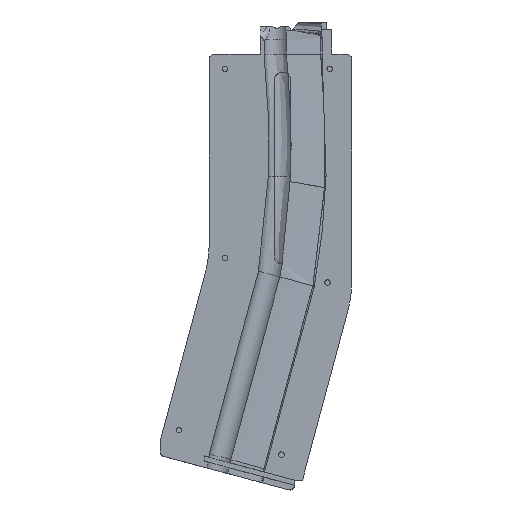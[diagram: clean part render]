
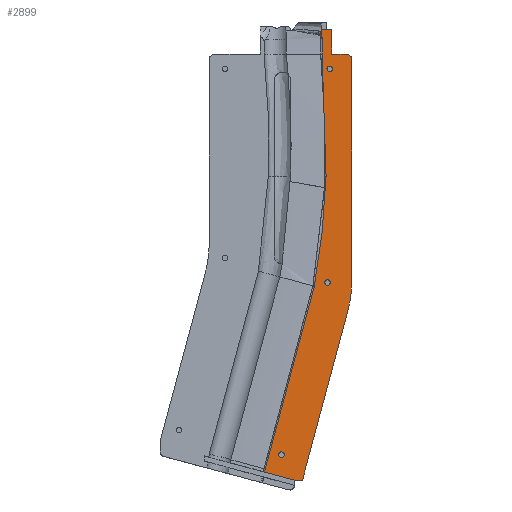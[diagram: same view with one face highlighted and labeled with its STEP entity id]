
A CAD part, front view. The second image highlights one B-rep face of the part: STEP entity #2899.
In plain terms, the highlighted planar face has unit normal (0, -1, 0).
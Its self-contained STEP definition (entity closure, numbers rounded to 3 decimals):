
#31=FACE_BOUND('',#755,.T.);
#32=FACE_BOUND('',#756,.T.);
#33=FACE_BOUND('',#757,.T.);
#140=LINE('',#5888,#327);
#141=LINE('',#5890,#328);
#142=LINE('',#5892,#329);
#143=LINE('',#5896,#330);
#144=LINE('',#5908,#331);
#145=LINE('',#5910,#332);
#146=LINE('',#5919,#333);
#147=LINE('',#5921,#334);
#148=LINE('',#5923,#335);
#149=LINE('',#5925,#336);
#150=LINE('',#5929,#337);
#151=LINE('',#5932,#338);
#327=VECTOR('',#3531,10.);
#328=VECTOR('',#3532,10.);
#329=VECTOR('',#3533,10.);
#330=VECTOR('',#3536,10.);
#331=VECTOR('',#3537,10.);
#332=VECTOR('',#3538,10.);
#333=VECTOR('',#3539,10.);
#334=VECTOR('',#3540,10.);
#335=VECTOR('',#3541,10.);
#336=VECTOR('',#3542,10.);
#337=VECTOR('',#3545,10.);
#338=VECTOR('',#3548,10.);
#470=PLANE('',#3127);
#571=FACE_OUTER_BOUND('',#754,.T.);
#754=EDGE_LOOP('',(#2173,#2174,#2175,#2176,#2177,#2178,#2179,#2180,#2181,
#2182,#2183,#2184,#2185,#2186,#2187,#2188,#2189,#2190));
#755=EDGE_LOOP('',(#2191));
#756=EDGE_LOOP('',(#2192));
#757=EDGE_LOOP('',(#2193));
#900=CIRCLE('',#3072,1.25);
#921=CIRCLE('',#3128,2.);
#922=CIRCLE('',#3129,50.);
#923=CIRCLE('',#3130,2.5);
#924=CIRCLE('',#3131,1.25);
#925=CIRCLE('',#3132,1.25);
#1108=B_SPLINE_CURVE_WITH_KNOTS('',3,(#5898,#5899,#5900,#5901),
 .UNSPECIFIED.,.F.,.F.,(4,4),(-5.507,0.),.UNSPECIFIED.);
#1109=B_SPLINE_CURVE_WITH_KNOTS('',3,(#5903,#5904,#5905,#5906),
 .UNSPECIFIED.,.F.,.F.,(4,4),(-4.958,0.),.UNSPECIFIED.);
#1110=B_SPLINE_CURVE_WITH_KNOTS('',3,(#5912,#5913,#5914,#5915,#5916,#5917),
 .UNSPECIFIED.,.F.,.F.,(4,2,4),(-0.151,-0.075,
0.),.UNSPECIFIED.);
#1230=VERTEX_POINT('',#5105);
#1302=VERTEX_POINT('',#5886);
#1303=VERTEX_POINT('',#5887);
#1304=VERTEX_POINT('',#5889);
#1305=VERTEX_POINT('',#5891);
#1306=VERTEX_POINT('',#5893);
#1307=VERTEX_POINT('',#5895);
#1308=VERTEX_POINT('',#5897);
#1309=VERTEX_POINT('',#5902);
#1310=VERTEX_POINT('',#5907);
#1311=VERTEX_POINT('',#5909);
#1312=VERTEX_POINT('',#5911);
#1313=VERTEX_POINT('',#5918);
#1314=VERTEX_POINT('',#5920);
#1315=VERTEX_POINT('',#5922);
#1316=VERTEX_POINT('',#5924);
#1317=VERTEX_POINT('',#5926);
#1318=VERTEX_POINT('',#5928);
#1319=VERTEX_POINT('',#5930);
#1320=VERTEX_POINT('',#5933);
#1321=VERTEX_POINT('',#5935);
#1531=EDGE_CURVE('',#1230,#1230,#900,.T.);
#1633=EDGE_CURVE('',#1302,#1303,#140,.T.);
#1634=EDGE_CURVE('',#1304,#1302,#141,.T.);
#1635=EDGE_CURVE('',#1305,#1304,#142,.T.);
#1636=EDGE_CURVE('',#1306,#1305,#921,.T.);
#1637=EDGE_CURVE('',#1307,#1306,#143,.T.);
#1638=EDGE_CURVE('',#1308,#1307,#1108,.T.);
#1639=EDGE_CURVE('',#1309,#1308,#1109,.T.);
#1640=EDGE_CURVE('',#1309,#1310,#144,.T.);
#1641=EDGE_CURVE('',#1310,#1311,#145,.T.);
#1642=EDGE_CURVE('',#1312,#1311,#1110,.T.);
#1643=EDGE_CURVE('',#1313,#1312,#146,.T.);
#1644=EDGE_CURVE('',#1314,#1313,#147,.T.);
#1645=EDGE_CURVE('',#1315,#1314,#148,.T.);
#1646=EDGE_CURVE('',#1315,#1316,#149,.T.);
#1647=EDGE_CURVE('',#1317,#1316,#922,.F.);
#1648=EDGE_CURVE('',#1318,#1317,#150,.T.);
#1649=EDGE_CURVE('',#1319,#1318,#923,.T.);
#1650=EDGE_CURVE('',#1303,#1319,#151,.T.);
#1651=EDGE_CURVE('',#1320,#1320,#924,.T.);
#1652=EDGE_CURVE('',#1321,#1321,#925,.T.);
#2173=ORIENTED_EDGE('',*,*,#1633,.F.);
#2174=ORIENTED_EDGE('',*,*,#1634,.F.);
#2175=ORIENTED_EDGE('',*,*,#1635,.F.);
#2176=ORIENTED_EDGE('',*,*,#1636,.F.);
#2177=ORIENTED_EDGE('',*,*,#1637,.F.);
#2178=ORIENTED_EDGE('',*,*,#1638,.F.);
#2179=ORIENTED_EDGE('',*,*,#1639,.F.);
#2180=ORIENTED_EDGE('',*,*,#1640,.T.);
#2181=ORIENTED_EDGE('',*,*,#1641,.T.);
#2182=ORIENTED_EDGE('',*,*,#1642,.F.);
#2183=ORIENTED_EDGE('',*,*,#1643,.F.);
#2184=ORIENTED_EDGE('',*,*,#1644,.F.);
#2185=ORIENTED_EDGE('',*,*,#1645,.F.);
#2186=ORIENTED_EDGE('',*,*,#1646,.T.);
#2187=ORIENTED_EDGE('',*,*,#1647,.F.);
#2188=ORIENTED_EDGE('',*,*,#1648,.F.);
#2189=ORIENTED_EDGE('',*,*,#1649,.F.);
#2190=ORIENTED_EDGE('',*,*,#1650,.F.);
#2191=ORIENTED_EDGE('',*,*,#1651,.F.);
#2192=ORIENTED_EDGE('',*,*,#1531,.F.);
#2193=ORIENTED_EDGE('',*,*,#1652,.F.);
#2899=ADVANCED_FACE('',(#571,#31,#32,#33),#470,.F.);
#3072=AXIS2_PLACEMENT_3D('',#5106,#3375,#3376);
#3127=AXIS2_PLACEMENT_3D('',#5885,#3529,#3530);
#3128=AXIS2_PLACEMENT_3D('',#5894,#3534,#3535);
#3129=AXIS2_PLACEMENT_3D('',#5927,#3543,#3544);
#3130=AXIS2_PLACEMENT_3D('',#5931,#3546,#3547);
#3131=AXIS2_PLACEMENT_3D('',#5934,#3549,#3550);
#3132=AXIS2_PLACEMENT_3D('',#5936,#3551,#3552);
#3375=DIRECTION('center_axis',(0.,-1.,0.));
#3376=DIRECTION('ref_axis',(1.,0.,0.));
#3529=DIRECTION('center_axis',(0.,1.,0.));
#3530=DIRECTION('ref_axis',(0.,0.,1.));
#3531=DIRECTION('',(0.,0.,-1.));
#3532=DIRECTION('',(1.,0.,0.));
#3533=DIRECTION('',(0.,0.,1.));
#3534=DIRECTION('center_axis',(0.,-1.,0.));
#3535=DIRECTION('ref_axis',(0.77,0.,0.639));
#3536=DIRECTION('',(0.,0.,1.));
#3537=DIRECTION('',(-0.259,0.,-0.966));
#3538=DIRECTION('',(-0.966,0.,0.259));
#3539=DIRECTION('',(-0.966,0.,0.259));
#3540=DIRECTION('',(-1.,0.,0.));
#3541=DIRECTION('',(0.,0.,-1.));
#3542=DIRECTION('',(0.259,0.,0.966));
#3543=DIRECTION('center_axis',(0.,-1.,0.));
#3544=DIRECTION('ref_axis',(0.991,0.,-0.131));
#3545=DIRECTION('',(0.,0.,-1.));
#3546=DIRECTION('center_axis',(0.,1.,0.));
#3547=DIRECTION('ref_axis',(0.707,0.,0.707));
#3548=DIRECTION('',(1.,0.,0.));
#3549=DIRECTION('center_axis',(0.,-1.,0.));
#3550=DIRECTION('ref_axis',(1.,0.,0.));
#3551=DIRECTION('center_axis',(0.,-1.,0.));
#3552=DIRECTION('ref_axis',(1.,0.,0.));
#5105=CARTESIAN_POINT('',(388.993,-27.877,26.866));
#5106=CARTESIAN_POINT('Origin',(390.243,-27.877,26.866));
#5885=CARTESIAN_POINT('Origin',(357.119,-27.877,-57.186));
#5886=CARTESIAN_POINT('',(391.124,-27.877,44.387));
#5887=CARTESIAN_POINT('',(391.124,-27.877,33.487));
#5888=CARTESIAN_POINT('',(391.124,-27.877,-9.624));
#5889=CARTESIAN_POINT('',(386.532,-27.877,44.387));
#5890=CARTESIAN_POINT('',(374.121,-27.877,44.387));
#5891=CARTESIAN_POINT('',(386.532,-27.877,41.603));
#5892=CARTESIAN_POINT('',(386.532,-27.877,-6.528));
#5893=CARTESIAN_POINT('',(386.804,-27.877,40.597));
#5894=CARTESIAN_POINT('Origin',(384.804,-27.877,40.597));
#5895=CARTESIAN_POINT('',(386.804,-27.877,33.487));
#5896=CARTESIAN_POINT('',(386.804,-27.877,-8.593));
#5897=CARTESIAN_POINT('',(388.588,-27.877,-21.513));
#5898=CARTESIAN_POINT('Ctrl Pts',(388.588,-27.877,-21.513));
#5899=CARTESIAN_POINT('Ctrl Pts',(389.224,-27.877,-3.789));
#5900=CARTESIAN_POINT('Ctrl Pts',(388.616,-27.877,14.51));
#5901=CARTESIAN_POINT('Ctrl Pts',(386.804,-27.877,33.487));
#5902=CARTESIAN_POINT('',(383.307,-27.877,-70.728));
#5903=CARTESIAN_POINT('Ctrl Pts',(383.307,-27.877,-70.728));
#5904=CARTESIAN_POINT('Ctrl Pts',(386.251,-27.877,-54.706));
#5905=CARTESIAN_POINT('Ctrl Pts',(387.983,-27.877,-38.366));
#5906=CARTESIAN_POINT('Ctrl Pts',(388.588,-27.877,-21.513));
#5907=CARTESIAN_POINT('',(361.333,-27.877,-152.735));
#5908=CARTESIAN_POINT('',(383.307,-27.877,-70.728));
#5909=CARTESIAN_POINT('',(361.307,-27.877,-152.728));
#5910=CARTESIAN_POINT('',(337.591,-27.877,-146.373));
#5911=CARTESIAN_POINT('',(361.031,-27.877,-154.21));
#5912=CARTESIAN_POINT('Ctrl Pts',(361.031,-27.877,-154.21));
#5913=CARTESIAN_POINT('Ctrl Pts',(361.078,-27.877,-153.963));
#5914=CARTESIAN_POINT('Ctrl Pts',(361.124,-27.877,-153.716));
#5915=CARTESIAN_POINT('Ctrl Pts',(361.216,-27.877,-153.222));
#5916=CARTESIAN_POINT('Ctrl Pts',(361.262,-27.877,-152.975));
#5917=CARTESIAN_POINT('Ctrl Pts',(361.307,-27.877,-152.728));
#5918=CARTESIAN_POINT('',(375.09,-27.877,-157.977));
#5919=CARTESIAN_POINT('',(344.973,-27.877,-149.907));
#5920=CARTESIAN_POINT('',(378.124,-27.877,-157.977));
#5921=CARTESIAN_POINT('',(365.621,-27.877,-157.977));
#5922=CARTESIAN_POINT('',(378.124,-27.877,-157.339));
#5923=CARTESIAN_POINT('',(378.124,-27.877,-52.849));
#5924=CARTESIAN_POINT('',(398.42,-27.877,-81.592));
#5925=CARTESIAN_POINT('',(406.559,-27.877,-51.218));
#5926=CARTESIAN_POINT('',(400.124,-27.877,-68.651));
#5927=CARTESIAN_POINT('Origin',(350.124,-27.877,-68.651));
#5928=CARTESIAN_POINT('',(400.124,-27.877,30.987));
#5929=CARTESIAN_POINT('',(400.124,-27.877,-11.849));
#5930=CARTESIAN_POINT('',(397.624,-27.877,33.487));
#5931=CARTESIAN_POINT('Origin',(397.624,-27.877,30.987));
#5932=CARTESIAN_POINT('',(373.141,-27.877,33.487));
#5933=CARTESIAN_POINT('',(367.287,-27.877,-146.408));
#5934=CARTESIAN_POINT('Origin',(368.537,-27.877,-146.408));
#5935=CARTESIAN_POINT('',(387.993,-27.877,-69.134));
#5936=CARTESIAN_POINT('Origin',(389.243,-27.877,-69.134));
